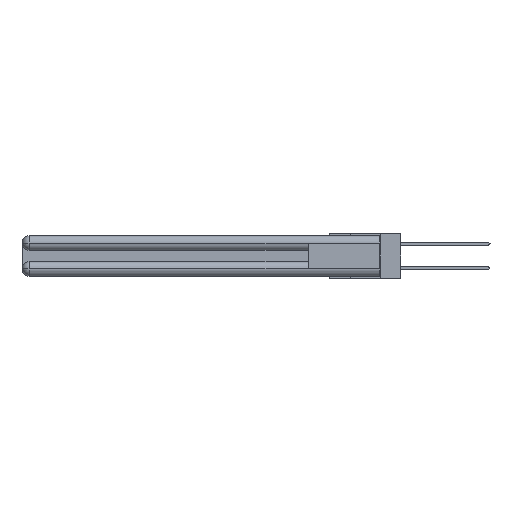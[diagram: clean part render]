
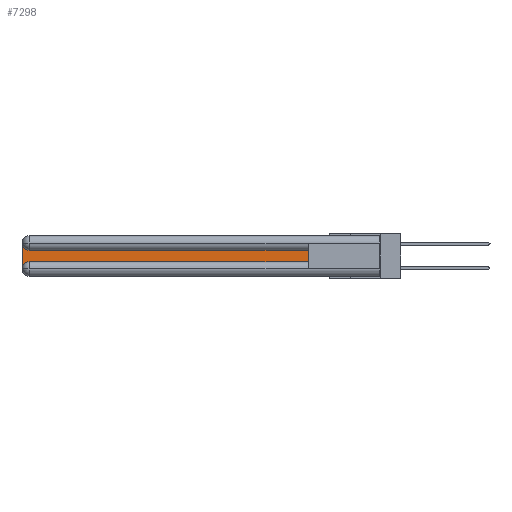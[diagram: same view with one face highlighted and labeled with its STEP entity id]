
A CAD part, left-side view. The second image highlights one B-rep face of the part: STEP entity #7298.
In plain terms, the highlighted planar face has unit normal (-1, 0, 0).
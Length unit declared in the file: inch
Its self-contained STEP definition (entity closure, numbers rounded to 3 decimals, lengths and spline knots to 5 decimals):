
#1407 = CIRCLE ( 'NONE', #29234, 0.06 ) ;
#1445 = VECTOR ( 'NONE', #13489, 39.37008 ) ;
#2245 = CARTESIAN_POINT ( 'NONE',  ( 0.075, 2.94, -0.1225 ) ) ;
#2307 = LINE ( 'NONE', #8548, #24024 ) ;
#2387 = CARTESIAN_POINT ( 'NONE',  ( 0.075, 0.6, -0.1225 ) ) ;
#4522 = CARTESIAN_POINT ( 'NONE',  ( 0.075, 3., -0.2175 ) ) ;
#5229 = LINE ( 'NONE', #21064, #1445 ) ;
#5385 = EDGE_CURVE ( 'NONE', #8953, #16558, #1407, .T. ) ;
#5411 = FACE_OUTER_BOUND ( 'NONE', #9111, .T. ) ;
#5799 = ORIENTED_EDGE ( 'NONE', *, *, #25416, .T. ) ;
#5950 = EDGE_CURVE ( 'NONE', #6583, #8953, #26132, .T. ) ;
#6033 = DIRECTION ( 'NONE',  ( 0., 0., -1. ) ) ;
#6247 = CARTESIAN_POINT ( 'NONE',  ( 0.075, 0.6, -0.2175 ) ) ;
#6583 = VERTEX_POINT ( 'NONE', #19857 ) ;
#7298 = ADVANCED_FACE ( 'NONE', ( #5411 ), #8147, .F. ) ;
#8147 = PLANE ( 'NONE',  #22815 ) ;
#8356 = CARTESIAN_POINT ( 'NONE',  ( 0.075, 2.94, -0.2775 ) ) ;
#8548 = CARTESIAN_POINT ( 'NONE',  ( 0.075, 0.6, -0.2175 ) ) ;
#8758 = DIRECTION ( 'NONE',  ( 0., -1., 0. ) ) ;
#8953 = VERTEX_POINT ( 'NONE', #13099 ) ;
#9111 = EDGE_LOOP ( 'NONE', ( #30412, #25908, #28258, #12313, #5799, #20586 ) ) ;
#10028 = EDGE_CURVE ( 'NONE', #22015, #6583, #18495, .T. ) ;
#11753 = CARTESIAN_POINT ( 'NONE',  ( 0.075, 2.94, -0.0625 ) ) ;
#12313 = ORIENTED_EDGE ( 'NONE', *, *, #5385, .T. ) ;
#13099 = CARTESIAN_POINT ( 'NONE',  ( 0.075, 3., -0.2775 ) ) ;
#13398 = CARTESIAN_POINT ( 'NONE',  ( 0.075, 3., -0.1225 ) ) ;
#13460 = EDGE_CURVE ( 'NONE', #21370, #13857, #5229, .T. ) ;
#13489 = DIRECTION ( 'NONE',  ( 0., 0., 1. ) ) ;
#13857 = VERTEX_POINT ( 'NONE', #18341 ) ;
#14423 = DIRECTION ( 'NONE',  ( 0., 0., -1. ) ) ;
#15701 = LINE ( 'NONE', #2387, #25589 ) ;
#16558 = VERTEX_POINT ( 'NONE', #23808 ) ;
#17004 = DIRECTION ( 'NONE',  ( 1., 0., 0. ) ) ;
#18341 = CARTESIAN_POINT ( 'NONE',  ( 0.075, 0.6, -0.1225 ) ) ;
#18495 = CIRCLE ( 'NONE', #24057, 0.06 ) ;
#19857 = CARTESIAN_POINT ( 'NONE',  ( 0.075, 3., -0.0625 ) ) ;
#20346 = DIRECTION ( 'NONE',  ( 0., 0., -1. ) ) ;
#20586 = ORIENTED_EDGE ( 'NONE', *, *, #13460, .T. ) ;
#20655 = DIRECTION ( 'NONE',  ( 1., 0., 0. ) ) ;
#21064 = CARTESIAN_POINT ( 'NONE',  ( 0.075, 0.6, -0.2175 ) ) ;
#21370 = VERTEX_POINT ( 'NONE', #6247 ) ;
#21570 = DIRECTION ( 'NONE',  ( 0., 0., -1. ) ) ;
#21602 = EDGE_CURVE ( 'NONE', #13857, #22015, #15701, .T. ) ;
#21883 = DIRECTION ( 'NONE',  ( 0., 1., 0. ) ) ;
#22015 = VERTEX_POINT ( 'NONE', #2245 ) ;
#22815 = AXIS2_PLACEMENT_3D ( 'NONE', #13398, #30311, #20346 ) ;
#23808 = CARTESIAN_POINT ( 'NONE',  ( 0.075, 2.94, -0.2175 ) ) ;
#24024 = VECTOR ( 'NONE', #8758, 39.37008 ) ;
#24057 = AXIS2_PLACEMENT_3D ( 'NONE', #11753, #17004, #14423 ) ;
#25416 = EDGE_CURVE ( 'NONE', #16558, #21370, #2307, .T. ) ;
#25589 = VECTOR ( 'NONE', #21883, 39.37008 ) ;
#25908 = ORIENTED_EDGE ( 'NONE', *, *, #10028, .T. ) ;
#26132 = LINE ( 'NONE', #4522, #28754 ) ;
#28258 = ORIENTED_EDGE ( 'NONE', *, *, #5950, .T. ) ;
#28754 = VECTOR ( 'NONE', #21570, 39.37008 ) ;
#29234 = AXIS2_PLACEMENT_3D ( 'NONE', #8356, #20655, #6033 ) ;
#30311 = DIRECTION ( 'NONE',  ( 1., 0., 0. ) ) ;
#30412 = ORIENTED_EDGE ( 'NONE', *, *, #21602, .T. ) ;
